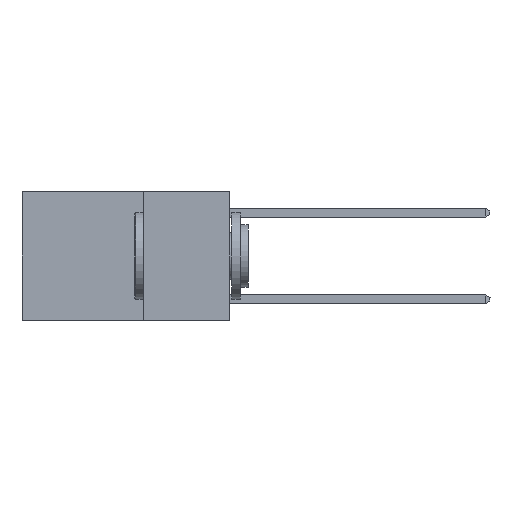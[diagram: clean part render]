
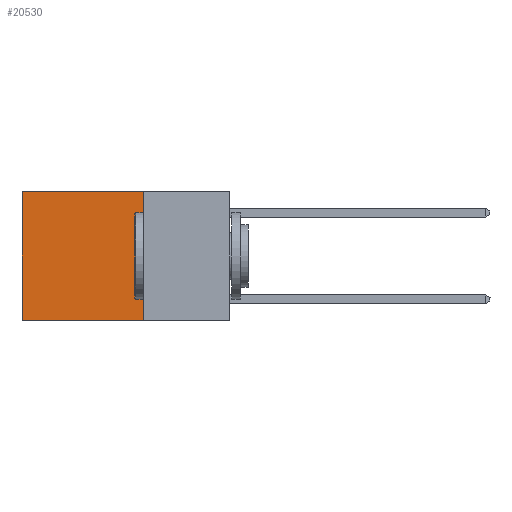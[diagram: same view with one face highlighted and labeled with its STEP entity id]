
A CAD part, left-side view. The second image highlights one B-rep face of the part: STEP entity #20530.
In plain terms, the highlighted planar face has unit normal (-1, 0, 0).
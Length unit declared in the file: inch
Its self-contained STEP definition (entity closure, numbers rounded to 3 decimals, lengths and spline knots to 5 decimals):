
#1600 = CARTESIAN_POINT ( 'NONE',  ( 0.2625, 0.25, 0. ) ) ;
#1698 = VERTEX_POINT ( 'NONE', #22064 ) ;
#1856 = ORIENTED_EDGE ( 'NONE', *, *, #22655, .F. ) ;
#2079 = LINE ( 'NONE', #20897, #20258 ) ;
#2386 = EDGE_LOOP ( 'NONE', ( #3721, #4868, #1856, #5549 ) ) ;
#2481 = CARTESIAN_POINT ( 'NONE',  ( 0.2625, 0.6, -0.37 ) ) ;
#3721 = ORIENTED_EDGE ( 'NONE', *, *, #19508, .T. ) ;
#4516 = VERTEX_POINT ( 'NONE', #2481 ) ;
#4868 = ORIENTED_EDGE ( 'NONE', *, *, #5885, .F. ) ;
#5540 = EDGE_CURVE ( 'NONE', #14036, #11032, #2079, .T. ) ;
#5549 = ORIENTED_EDGE ( 'NONE', *, *, #5540, .T. ) ;
#5885 = EDGE_CURVE ( 'NONE', #1698, #4516, #14321, .T. ) ;
#8427 = CARTESIAN_POINT ( 'NONE',  ( 0.2625, 0.25, 0. ) ) ;
#9043 = DIRECTION ( 'NONE',  ( 1., 0., 0. ) ) ;
#10669 = VECTOR ( 'NONE', #17040, 39.37008 ) ;
#11032 = VERTEX_POINT ( 'NONE', #14187 ) ;
#11216 = LINE ( 'NONE', #11782, #10669 ) ;
#11782 = CARTESIAN_POINT ( 'NONE',  ( 0.2625, 0.6, 0. ) ) ;
#12307 = DIRECTION ( 'NONE',  ( 0., 0., -1. ) ) ;
#14036 = VERTEX_POINT ( 'NONE', #8427 ) ;
#14187 = CARTESIAN_POINT ( 'NONE',  ( 0.2625, 0.6, 0. ) ) ;
#14193 = FACE_OUTER_BOUND ( 'NONE', #2386, .T. ) ;
#14279 = LINE ( 'NONE', #1600, #17792 ) ;
#14321 = LINE ( 'NONE', #18192, #18375 ) ;
#16526 = DIRECTION ( 'NONE',  ( 0., 1., 0. ) ) ;
#17040 = DIRECTION ( 'NONE',  ( 0., 0., -1. ) ) ;
#17792 = VECTOR ( 'NONE', #12307, 39.37008 ) ;
#18192 = CARTESIAN_POINT ( 'NONE',  ( 0.2625, 0.25, -0.37 ) ) ;
#18375 = VECTOR ( 'NONE', #16526, 39.37008 ) ;
#19239 = DIRECTION ( 'NONE',  ( 0., 1., 0. ) ) ;
#19477 = CARTESIAN_POINT ( 'NONE',  ( 0.2625, 0.25, 0. ) ) ;
#19508 = EDGE_CURVE ( 'NONE', #11032, #4516, #11216, .T. ) ;
#19525 = AXIS2_PLACEMENT_3D ( 'NONE', #19477, #9043, #21212 ) ;
#20258 = VECTOR ( 'NONE', #19239, 39.37008 ) ;
#20530 = ADVANCED_FACE ( 'NONE', ( #14193 ), #22882, .F. ) ;
#20897 = CARTESIAN_POINT ( 'NONE',  ( 0.2625, 0.25, 0. ) ) ;
#21212 = DIRECTION ( 'NONE',  ( 0., 0., -1. ) ) ;
#22064 = CARTESIAN_POINT ( 'NONE',  ( 0.2625, 0.25, -0.37 ) ) ;
#22655 = EDGE_CURVE ( 'NONE', #14036, #1698, #14279, .T. ) ;
#22882 = PLANE ( 'NONE',  #19525 ) ;
